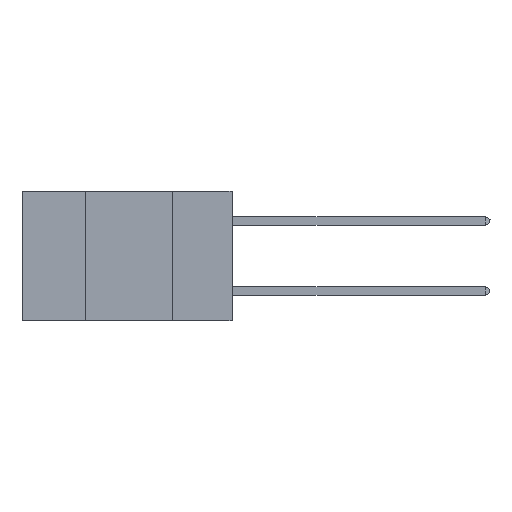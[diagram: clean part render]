
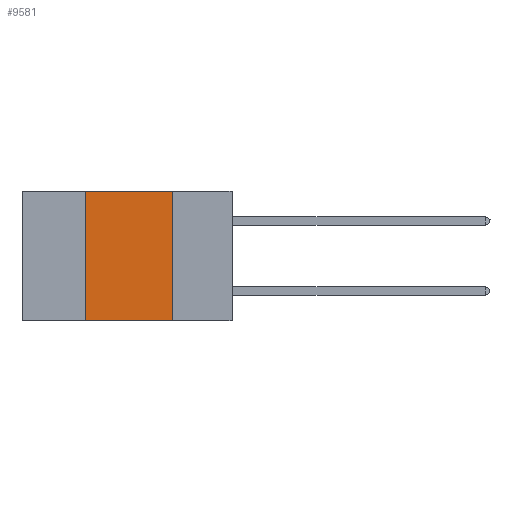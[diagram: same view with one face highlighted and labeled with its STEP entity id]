
A CAD part, left-side view. The second image highlights one B-rep face of the part: STEP entity #9581.
In plain terms, the highlighted planar face has unit normal (-1, 0, 0).
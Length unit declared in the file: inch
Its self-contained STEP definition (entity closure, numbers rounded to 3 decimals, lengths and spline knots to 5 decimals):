
#593 = LINE ( 'NONE', #24459, #9776 ) ;
#1507 = LINE ( 'NONE', #3467, #9296 ) ;
#2558 = EDGE_CURVE ( 'NONE', #12967, #8790, #22082, .T. ) ;
#3467 = CARTESIAN_POINT ( 'NONE',  ( 0., 0.6, 0. ) ) ;
#3562 = PLANE ( 'NONE',  #7998 ) ;
#3678 = ORIENTED_EDGE ( 'NONE', *, *, #23576, .T. ) ;
#6089 = ORIENTED_EDGE ( 'NONE', *, *, #15810, .F. ) ;
#6614 = DIRECTION ( 'NONE',  ( 0., -1., 0. ) ) ;
#7119 = CARTESIAN_POINT ( 'NONE',  ( 0., 0.42, 0. ) ) ;
#7942 = CARTESIAN_POINT ( 'NONE',  ( 0., 0.17, -0.37 ) ) ;
#7998 = AXIS2_PLACEMENT_3D ( 'NONE', #25438, #16086, #15573 ) ;
#8790 = VERTEX_POINT ( 'NONE', #7942 ) ;
#9296 = VECTOR ( 'NONE', #14877, 39.37008 ) ;
#9581 = ADVANCED_FACE ( 'NONE', ( #21663 ), #3562, .F. ) ;
#9776 = VECTOR ( 'NONE', #6614, 39.37008 ) ;
#10497 = VERTEX_POINT ( 'NONE', #12774 ) ;
#11648 = CARTESIAN_POINT ( 'NONE',  ( 0., 0.42, 0. ) ) ;
#12774 = CARTESIAN_POINT ( 'NONE',  ( 0., 0.42, -0.37 ) ) ;
#12967 = VERTEX_POINT ( 'NONE', #22658 ) ;
#14877 = DIRECTION ( 'NONE',  ( 0., -1., 0. ) ) ;
#15566 = LINE ( 'NONE', #11648, #21857 ) ;
#15573 = DIRECTION ( 'NONE',  ( 0., 0., -1. ) ) ;
#15810 = EDGE_CURVE ( 'NONE', #10497, #23708, #15566, .T. ) ;
#16086 = DIRECTION ( 'NONE',  ( 1., 0., 0. ) ) ;
#17747 = EDGE_CURVE ( 'NONE', #23708, #12967, #1507, .T. ) ;
#18298 = DIRECTION ( 'NONE',  ( 0., 0., -1. ) ) ;
#19567 = DIRECTION ( 'NONE',  ( 0., 0., 1. ) ) ;
#21663 = FACE_OUTER_BOUND ( 'NONE', #23207, .T. ) ;
#21857 = VECTOR ( 'NONE', #19567, 39.37008 ) ;
#22082 = LINE ( 'NONE', #22216, #25112 ) ;
#22216 = CARTESIAN_POINT ( 'NONE',  ( 0., 0.17, 0. ) ) ;
#22658 = CARTESIAN_POINT ( 'NONE',  ( 0., 0.17, 0. ) ) ;
#23207 = EDGE_LOOP ( 'NONE', ( #24982, #23852, #6089, #3678 ) ) ;
#23576 = EDGE_CURVE ( 'NONE', #10497, #8790, #593, .T. ) ;
#23708 = VERTEX_POINT ( 'NONE', #7119 ) ;
#23852 = ORIENTED_EDGE ( 'NONE', *, *, #17747, .F. ) ;
#24459 = CARTESIAN_POINT ( 'NONE',  ( 0., 0.6, -0.37 ) ) ;
#24982 = ORIENTED_EDGE ( 'NONE', *, *, #2558, .F. ) ;
#25112 = VECTOR ( 'NONE', #18298, 39.37008 ) ;
#25438 = CARTESIAN_POINT ( 'NONE',  ( 0., 0.6, 0. ) ) ;
